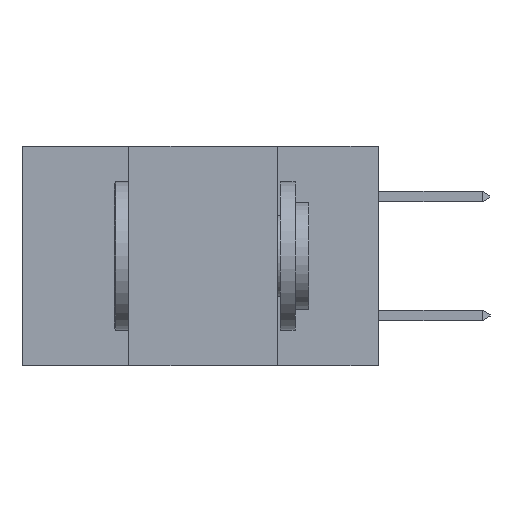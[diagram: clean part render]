
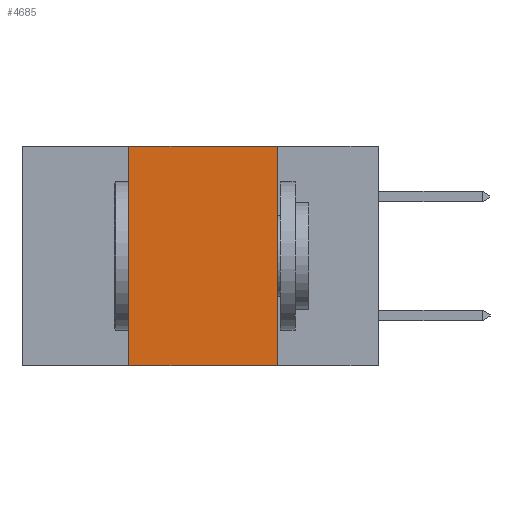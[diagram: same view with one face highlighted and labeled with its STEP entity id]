
A CAD part, left-side view. The second image highlights one B-rep face of the part: STEP entity #4685.
In plain terms, the highlighted planar face has unit normal (-1, 0, 0).
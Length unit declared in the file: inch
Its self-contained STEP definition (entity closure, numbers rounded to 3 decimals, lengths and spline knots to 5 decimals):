
#1086 = VERTEX_POINT ( 'NONE', #12628 ) ;
#1543 = LINE ( 'NONE', #6818, #13203 ) ;
#2965 = DIRECTION ( 'NONE',  ( 0., 0., -1. ) ) ;
#3143 = DIRECTION ( 'NONE',  ( 1., 0., 0. ) ) ;
#3236 = EDGE_LOOP ( 'NONE', ( #12508, #6251, #8278, #5121 ) ) ;
#3305 = CARTESIAN_POINT ( 'NONE',  ( 0., 0.6, 0. ) ) ;
#3319 = FACE_OUTER_BOUND ( 'NONE', #3236, .T. ) ;
#4055 = PLANE ( 'NONE',  #5213 ) ;
#4369 = DIRECTION ( 'NONE',  ( 0., 0., 1. ) ) ;
#4388 = CARTESIAN_POINT ( 'NONE',  ( 0., 0.17, -0.37 ) ) ;
#4474 = CARTESIAN_POINT ( 'NONE',  ( 0., 0.42, -0.37 ) ) ;
#4685 = ADVANCED_FACE ( 'NONE', ( #3319 ), #4055, .F. ) ;
#5121 = ORIENTED_EDGE ( 'NONE', *, *, #14521, .T. ) ;
#5213 = AXIS2_PLACEMENT_3D ( 'NONE', #3305, #3143, #2965 ) ;
#5717 = VERTEX_POINT ( 'NONE', #11121 ) ;
#5917 = VECTOR ( 'NONE', #4369, 39.37008 ) ;
#5983 = CARTESIAN_POINT ( 'NONE',  ( 0., 0.42, -0.37 ) ) ;
#6251 = ORIENTED_EDGE ( 'NONE', *, *, #11095, .F. ) ;
#6814 = DIRECTION ( 'NONE',  ( 0., 0., -1. ) ) ;
#6818 = CARTESIAN_POINT ( 'NONE',  ( 0., 0.17, -0.37 ) ) ;
#8278 = ORIENTED_EDGE ( 'NONE', *, *, #15271, .F. ) ;
#9567 = VECTOR ( 'NONE', #12090, 39.37008 ) ;
#9865 = VERTEX_POINT ( 'NONE', #5983 ) ;
#10642 = CARTESIAN_POINT ( 'NONE',  ( 0., 0.6, -0.37 ) ) ;
#11042 = DIRECTION ( 'NONE',  ( 0., -1., 0. ) ) ;
#11095 = EDGE_CURVE ( 'NONE', #1086, #5717, #12672, .T. ) ;
#11121 = CARTESIAN_POINT ( 'NONE',  ( 0., 0.17, 0. ) ) ;
#11299 = VECTOR ( 'NONE', #11042, 39.37008 ) ;
#11658 = LINE ( 'NONE', #10642, #11299 ) ;
#11813 = LINE ( 'NONE', #4474, #5917 ) ;
#12090 = DIRECTION ( 'NONE',  ( 0., -1., 0. ) ) ;
#12140 = EDGE_CURVE ( 'NONE', #5717, #12645, #1543, .T. ) ;
#12293 = CARTESIAN_POINT ( 'NONE',  ( 0., 0.6, 0. ) ) ;
#12508 = ORIENTED_EDGE ( 'NONE', *, *, #12140, .F. ) ;
#12628 = CARTESIAN_POINT ( 'NONE',  ( 0., 0.42, 0. ) ) ;
#12645 = VERTEX_POINT ( 'NONE', #4388 ) ;
#12672 = LINE ( 'NONE', #12293, #9567 ) ;
#13203 = VECTOR ( 'NONE', #6814, 39.37008 ) ;
#14521 = EDGE_CURVE ( 'NONE', #9865, #12645, #11658, .T. ) ;
#15271 = EDGE_CURVE ( 'NONE', #9865, #1086, #11813, .T. ) ;
